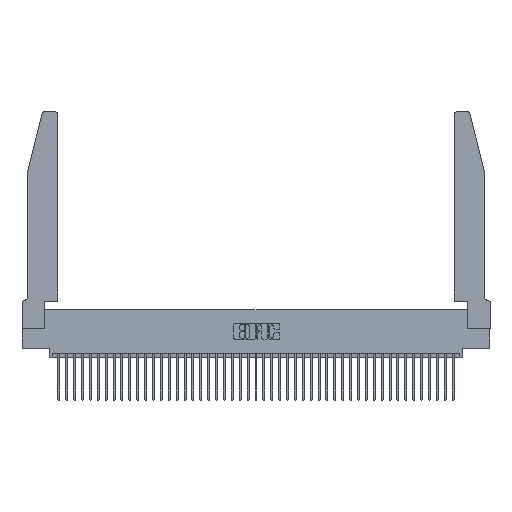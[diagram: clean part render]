
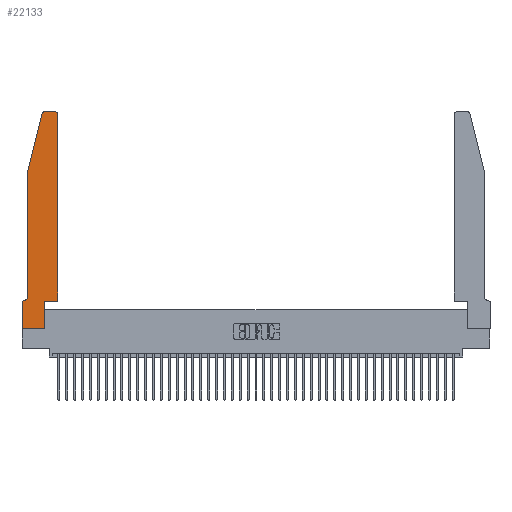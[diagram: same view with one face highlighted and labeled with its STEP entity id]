
A CAD part, top view. The second image highlights one B-rep face of the part: STEP entity #22133.
In plain terms, the highlighted planar face has unit normal (0, 0, 1).
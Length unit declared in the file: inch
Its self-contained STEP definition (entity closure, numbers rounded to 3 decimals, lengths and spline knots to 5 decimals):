
#463 = ORIENTED_EDGE ( 'NONE', *, *, #4480, .T. ) ;
#550 = VERTEX_POINT ( 'NONE', #10814 ) ;
#695 = CARTESIAN_POINT ( 'NONE',  ( 0.0755, 2., 0.37 ) ) ;
#775 = VECTOR ( 'NONE', #40345, 39.37008 ) ;
#841 = DIRECTION ( 'NONE',  ( 0., -1., 0. ) ) ;
#846 = CARTESIAN_POINT ( 'NONE',  ( 0.4505, 0.35, 0.37 ) ) ;
#1178 = VERTEX_POINT ( 'NONE', #33196 ) ;
#1591 = EDGE_CURVE ( 'NONE', #17533, #36983, #32619, .T. ) ;
#3700 = EDGE_CURVE ( 'NONE', #550, #30016, #43332, .T. ) ;
#3976 = CARTESIAN_POINT ( 'NONE',  ( 0.4505, 2.72, 0.37 ) ) ;
#4085 = CARTESIAN_POINT ( 'NONE',  ( 0.0755, 0.42, 0.37 ) ) ;
#4480 = EDGE_CURVE ( 'NONE', #28253, #10734, #10022, .T. ) ;
#4626 = ORIENTED_EDGE ( 'NONE', *, *, #20206, .T. ) ;
#4806 = LINE ( 'NONE', #10984, #20216 ) ;
#4844 = DIRECTION ( 'NONE',  ( 1., 0., 0. ) ) ;
#5337 = VERTEX_POINT ( 'NONE', #42918 ) ;
#5621 = VERTEX_POINT ( 'NONE', #7634 ) ;
#5817 = ORIENTED_EDGE ( 'NONE', *, *, #26148, .T. ) ;
#7219 = PLANE ( 'NONE',  #23538 ) ;
#7634 = CARTESIAN_POINT ( 'NONE',  ( 0., 0.35, 0.37 ) ) ;
#7646 = AXIS2_PLACEMENT_3D ( 'NONE', #35944, #26086, #25643 ) ;
#9946 = CIRCLE ( 'NONE', #21100, 0.07 ) ;
#10022 = LINE ( 'NONE', #28122, #36940 ) ;
#10734 = VERTEX_POINT ( 'NONE', #846 ) ;
#10814 = CARTESIAN_POINT ( 'NONE',  ( 0.4205, 2.75, 0.37 ) ) ;
#10841 = CARTESIAN_POINT ( 'NONE',  ( 0., 0., 0.37 ) ) ;
#10984 = CARTESIAN_POINT ( 'NONE',  ( 0.0755, 2., 0.37 ) ) ;
#11334 = EDGE_CURVE ( 'NONE', #1178, #28253, #33455, .T. ) ;
#11485 = VECTOR ( 'NONE', #36082, 39.37008 ) ;
#11639 = CIRCLE ( 'NONE', #15086, 0.03 ) ;
#12073 = EDGE_CURVE ( 'NONE', #5337, #17533, #4806, .T. ) ;
#12078 = VERTEX_POINT ( 'NONE', #3976 ) ;
#12946 = DIRECTION ( 'NONE',  ( 0., 0., -1. ) ) ;
#12948 = EDGE_CURVE ( 'NONE', #30016, #5337, #11639, .T. ) ;
#13119 = VECTOR ( 'NONE', #14522, 39.37008 ) ;
#13319 = CARTESIAN_POINT ( 'NONE',  ( 0., 0., 0.37 ) ) ;
#14428 = ORIENTED_EDGE ( 'NONE', *, *, #11334, .T. ) ;
#14522 = DIRECTION ( 'NONE',  ( 0., -1., 0. ) ) ;
#14917 = LINE ( 'NONE', #20670, #39702 ) ;
#15086 = AXIS2_PLACEMENT_3D ( 'NONE', #24846, #15240, #4844 ) ;
#15240 = DIRECTION ( 'NONE',  ( 0., 0., 1. ) ) ;
#15355 = EDGE_CURVE ( 'NONE', #18297, #5621, #28907, .T. ) ;
#15619 = EDGE_LOOP ( 'NONE', ( #24999, #25588, #31791, #27490, #19363, #43565, #5817, #4626, #14428, #463, #42195, #38963 ) ) ;
#16202 = DIRECTION ( 'NONE',  ( -1., 0., 0. ) ) ;
#16787 = CARTESIAN_POINT ( 'NONE',  ( 0., 0., 0.37 ) ) ;
#17039 = CARTESIAN_POINT ( 'NONE',  ( 0.2865, 0.35, 0.37 ) ) ;
#17226 = LINE ( 'NONE', #16787, #775 ) ;
#17365 = DIRECTION ( 'NONE',  ( -0.239, -0.971, 0. ) ) ;
#17533 = VERTEX_POINT ( 'NONE', #24531 ) ;
#18297 = VERTEX_POINT ( 'NONE', #21095 ) ;
#19029 = CARTESIAN_POINT ( 'NONE',  ( 0.284, 2.75, 0.37 ) ) ;
#19363 = ORIENTED_EDGE ( 'NONE', *, *, #37861, .T. ) ;
#20206 = EDGE_CURVE ( 'NONE', #43484, #1178, #17226, .T. ) ;
#20216 = VECTOR ( 'NONE', #17365, 39.37008 ) ;
#20425 = DIRECTION ( 'NONE',  ( 0., 1., 0. ) ) ;
#20670 = CARTESIAN_POINT ( 'NONE',  ( 0.4505, 0.35, 0.37 ) ) ;
#20706 = CARTESIAN_POINT ( 'NONE',  ( 0., 0.35, 0.37 ) ) ;
#21095 = CARTESIAN_POINT ( 'NONE',  ( 0.0055, 0.35, 0.37 ) ) ;
#21100 = AXIS2_PLACEMENT_3D ( 'NONE', #39197, #12946, #16202 ) ;
#21959 = EDGE_CURVE ( 'NONE', #10734, #12078, #14917, .T. ) ;
#22133 = ADVANCED_FACE ( 'NONE', ( #30183 ), #7219, .T. ) ;
#23538 = AXIS2_PLACEMENT_3D ( 'NONE', #20706, #34097, #26888 ) ;
#24531 = CARTESIAN_POINT ( 'NONE',  ( 0.0755, 2., 0.37 ) ) ;
#24759 = DIRECTION ( 'NONE',  ( 1., 0., 0. ) ) ;
#24846 = CARTESIAN_POINT ( 'NONE',  ( 0.284, 2.72, 0.37 ) ) ;
#24999 = ORIENTED_EDGE ( 'NONE', *, *, #3700, .T. ) ;
#25076 = CARTESIAN_POINT ( 'NONE',  ( 0.0755, 0.35, 0.37 ) ) ;
#25261 = VECTOR ( 'NONE', #841, 39.37008 ) ;
#25588 = ORIENTED_EDGE ( 'NONE', *, *, #12948, .T. ) ;
#25643 = DIRECTION ( 'NONE',  ( 1., 0., 0. ) ) ;
#26086 = DIRECTION ( 'NONE',  ( 0., 0., 1. ) ) ;
#26148 = EDGE_CURVE ( 'NONE', #5621, #43484, #41581, .T. ) ;
#26888 = DIRECTION ( 'NONE',  ( 1., 0., 0. ) ) ;
#27490 = ORIENTED_EDGE ( 'NONE', *, *, #1591, .T. ) ;
#27563 = DIRECTION ( 'NONE',  ( 0., 1., 0. ) ) ;
#28122 = CARTESIAN_POINT ( 'NONE',  ( 0.4505, 0.35, 0.37 ) ) ;
#28253 = VERTEX_POINT ( 'NONE', #33503 ) ;
#28907 = LINE ( 'NONE', #25076, #11485 ) ;
#30016 = VERTEX_POINT ( 'NONE', #19029 ) ;
#30183 = FACE_OUTER_BOUND ( 'NONE', #15619, .T. ) ;
#31791 = ORIENTED_EDGE ( 'NONE', *, *, #12073, .T. ) ;
#32619 = LINE ( 'NONE', #695, #25261 ) ;
#33196 = CARTESIAN_POINT ( 'NONE',  ( 0.2865, 0., 0.37 ) ) ;
#33455 = LINE ( 'NONE', #17039, #42969 ) ;
#33503 = CARTESIAN_POINT ( 'NONE',  ( 0.2865, 0.35, 0.37 ) ) ;
#34097 = DIRECTION ( 'NONE',  ( 0., 0., 1. ) ) ;
#34249 = EDGE_CURVE ( 'NONE', #12078, #550, #41145, .T. ) ;
#35944 = CARTESIAN_POINT ( 'NONE',  ( 0.4205, 2.72, 0.37 ) ) ;
#36082 = DIRECTION ( 'NONE',  ( -1., 0., 0. ) ) ;
#36940 = VECTOR ( 'NONE', #24759, 39.37008 ) ;
#36983 = VERTEX_POINT ( 'NONE', #4085 ) ;
#37861 = EDGE_CURVE ( 'NONE', #36983, #18297, #9946, .T. ) ;
#38405 = DIRECTION ( 'NONE',  ( -1., 0., 0. ) ) ;
#38590 = VECTOR ( 'NONE', #38405, 39.37008 ) ;
#38963 = ORIENTED_EDGE ( 'NONE', *, *, #34249, .T. ) ;
#39197 = CARTESIAN_POINT ( 'NONE',  ( 0.0055, 0.42, 0.37 ) ) ;
#39702 = VECTOR ( 'NONE', #27563, 39.37008 ) ;
#40345 = DIRECTION ( 'NONE',  ( 1., 0., 0. ) ) ;
#41145 = CIRCLE ( 'NONE', #7646, 0.03 ) ;
#41209 = CARTESIAN_POINT ( 'NONE',  ( 0.2605, 2.75, 0.37 ) ) ;
#41581 = LINE ( 'NONE', #10841, #13119 ) ;
#42195 = ORIENTED_EDGE ( 'NONE', *, *, #21959, .T. ) ;
#42918 = CARTESIAN_POINT ( 'NONE',  ( 0.25487, 2.72718, 0.37 ) ) ;
#42969 = VECTOR ( 'NONE', #20425, 39.37008 ) ;
#43332 = LINE ( 'NONE', #41209, #38590 ) ;
#43484 = VERTEX_POINT ( 'NONE', #13319 ) ;
#43565 = ORIENTED_EDGE ( 'NONE', *, *, #15355, .T. ) ;
